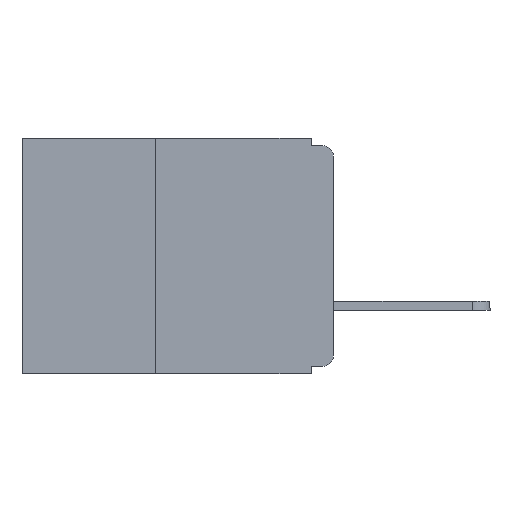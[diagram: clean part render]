
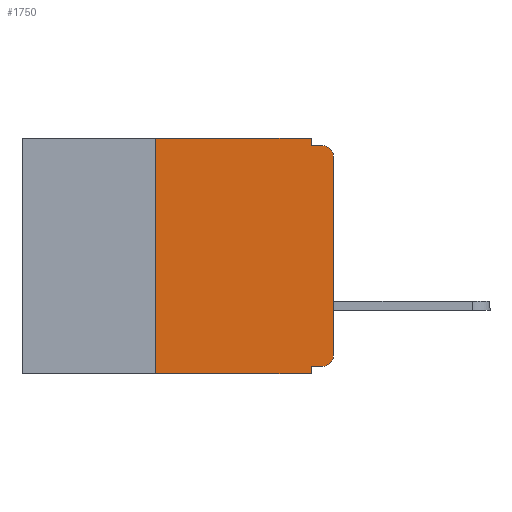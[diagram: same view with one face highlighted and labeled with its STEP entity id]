
A CAD part, left-side view. The second image highlights one B-rep face of the part: STEP entity #1750.
In plain terms, the highlighted planar face has unit normal (-1, 0, 0).
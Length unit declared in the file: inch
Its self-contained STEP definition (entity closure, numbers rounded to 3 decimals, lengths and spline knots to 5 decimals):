
#452 = CARTESIAN_POINT ( 'NONE',  ( 0., 0.031, 0. ) ) ;
#1750 = ADVANCED_FACE ( 'NONE', ( #9253 ), #13834, .F. ) ;
#2847 = EDGE_CURVE ( 'NONE', #5645, #4229, #3118, .T. ) ;
#3118 = CIRCLE ( 'NONE', #18012, 0.015 ) ;
#3281 = VERTEX_POINT ( 'NONE', #8255 ) ;
#3384 = ORIENTED_EDGE ( 'NONE', *, *, #25762, .F. ) ;
#3414 = DIRECTION ( 'NONE',  ( -1., 0., 0. ) ) ;
#4038 = VERTEX_POINT ( 'NONE', #6024 ) ;
#4229 = VERTEX_POINT ( 'NONE', #22526 ) ;
#5309 = VECTOR ( 'NONE', #12262, 39.37008 ) ;
#5504 = EDGE_LOOP ( 'NONE', ( #11152, #24888, #24540, #13641, #25946, #3384, #28102, #7116, #8626, #20961 ) ) ;
#5645 = VERTEX_POINT ( 'NONE', #16124 ) ;
#6024 = CARTESIAN_POINT ( 'NONE',  ( 0., 0.031, 0. ) ) ;
#6256 = VECTOR ( 'NONE', #16753, 39.37008 ) ;
#6316 = CARTESIAN_POINT ( 'NONE',  ( 0., 0.25, -0.33 ) ) ;
#6868 = CARTESIAN_POINT ( 'NONE',  ( 0., 0.437, 0. ) ) ;
#6939 = VERTEX_POINT ( 'NONE', #25939 ) ;
#6987 = LINE ( 'NONE', #23756, #6256 ) ;
#7116 = ORIENTED_EDGE ( 'NONE', *, *, #27860, .F. ) ;
#7436 = CIRCLE ( 'NONE', #28601, 0.015 ) ;
#7560 = VECTOR ( 'NONE', #28402, 39.37008 ) ;
#7600 = VERTEX_POINT ( 'NONE', #27231 ) ;
#7620 = VERTEX_POINT ( 'NONE', #15717 ) ;
#8001 = LINE ( 'NONE', #6316, #13425 ) ;
#8014 = DIRECTION ( 'NONE',  ( 0., 0., -1. ) ) ;
#8255 = CARTESIAN_POINT ( 'NONE',  ( 0., 0., -0.025 ) ) ;
#8626 = ORIENTED_EDGE ( 'NONE', *, *, #26238, .F. ) ;
#8899 = VECTOR ( 'NONE', #28273, 39.37008 ) ;
#9253 = FACE_OUTER_BOUND ( 'NONE', #5504, .T. ) ;
#9616 = EDGE_CURVE ( 'NONE', #24625, #13089, #23746, .T. ) ;
#11152 = ORIENTED_EDGE ( 'NONE', *, *, #16789, .T. ) ;
#11341 = CARTESIAN_POINT ( 'NONE',  ( 0., 0.031, -0.01 ) ) ;
#11606 = DIRECTION ( 'NONE',  ( 0., -1., 0. ) ) ;
#12262 = DIRECTION ( 'NONE',  ( 0., 0., -1. ) ) ;
#12718 = DIRECTION ( 'NONE',  ( 0., 1., 0. ) ) ;
#12784 = EDGE_CURVE ( 'NONE', #4038, #24625, #18439, .T. ) ;
#13089 = VERTEX_POINT ( 'NONE', #17900 ) ;
#13377 = VECTOR ( 'NONE', #29876, 39.37008 ) ;
#13425 = VECTOR ( 'NONE', #24902, 39.37008 ) ;
#13641 = ORIENTED_EDGE ( 'NONE', *, *, #12784, .F. ) ;
#13834 = PLANE ( 'NONE',  #20342 ) ;
#14919 = CARTESIAN_POINT ( 'NONE',  ( 0., 0., -0.32 ) ) ;
#15717 = CARTESIAN_POINT ( 'NONE',  ( 0., 0.25, 0. ) ) ;
#16014 = DIRECTION ( 'NONE',  ( -1., 0., 0. ) ) ;
#16124 = CARTESIAN_POINT ( 'NONE',  ( 0., 0.015, -0.32 ) ) ;
#16564 = EDGE_CURVE ( 'NONE', #7620, #4038, #26407, .T. ) ;
#16753 = DIRECTION ( 'NONE',  ( 0., -1., 0. ) ) ;
#16789 = EDGE_CURVE ( 'NONE', #4229, #3281, #26019, .T. ) ;
#17427 = CARTESIAN_POINT ( 'NONE',  ( 0., 0.015, -0.025 ) ) ;
#17900 = CARTESIAN_POINT ( 'NONE',  ( 0., 0.015, -0.01 ) ) ;
#18012 = AXIS2_PLACEMENT_3D ( 'NONE', #22515, #16014, #8014 ) ;
#18439 = LINE ( 'NONE', #452, #5309 ) ;
#18515 = EDGE_CURVE ( 'NONE', #3281, #13089, #7436, .T. ) ;
#18534 = VECTOR ( 'NONE', #12718, 39.37008 ) ;
#19364 = CARTESIAN_POINT ( 'NONE',  ( 0., 0.25, -0.33 ) ) ;
#19587 = EDGE_CURVE ( 'NONE', #24938, #6939, #6987, .T. ) ;
#19771 = DIRECTION ( 'NONE',  ( 0., 0., -1. ) ) ;
#20342 = AXIS2_PLACEMENT_3D ( 'NONE', #27712, #29252, #21802 ) ;
#20961 = ORIENTED_EDGE ( 'NONE', *, *, #2847, .T. ) ;
#21802 = DIRECTION ( 'NONE',  ( 0., 0., -1. ) ) ;
#22515 = CARTESIAN_POINT ( 'NONE',  ( 0., 0.015, -0.305 ) ) ;
#22526 = CARTESIAN_POINT ( 'NONE',  ( 0., 0., -0.305 ) ) ;
#23746 = LINE ( 'NONE', #29960, #29755 ) ;
#23756 = CARTESIAN_POINT ( 'NONE',  ( 0., 0.437, -0.33 ) ) ;
#24540 = ORIENTED_EDGE ( 'NONE', *, *, #9616, .F. ) ;
#24625 = VERTEX_POINT ( 'NONE', #11341 ) ;
#24694 = LINE ( 'NONE', #14919, #18534 ) ;
#24888 = ORIENTED_EDGE ( 'NONE', *, *, #18515, .T. ) ;
#24902 = DIRECTION ( 'NONE',  ( 0., 0., 1. ) ) ;
#24938 = VERTEX_POINT ( 'NONE', #19364 ) ;
#25762 = EDGE_CURVE ( 'NONE', #24938, #7620, #8001, .T. ) ;
#25939 = CARTESIAN_POINT ( 'NONE',  ( 0., 0.031, -0.33 ) ) ;
#25946 = ORIENTED_EDGE ( 'NONE', *, *, #16564, .F. ) ;
#25977 = CARTESIAN_POINT ( 'NONE',  ( 0., 0.031, -0.33 ) ) ;
#26019 = LINE ( 'NONE', #26103, #7560 ) ;
#26103 = CARTESIAN_POINT ( 'NONE',  ( 0., 0., 0. ) ) ;
#26238 = EDGE_CURVE ( 'NONE', #5645, #7600, #24694, .T. ) ;
#26407 = LINE ( 'NONE', #6868, #13377 ) ;
#27231 = CARTESIAN_POINT ( 'NONE',  ( 0., 0.031, -0.32 ) ) ;
#27316 = LINE ( 'NONE', #25977, #8899 ) ;
#27712 = CARTESIAN_POINT ( 'NONE',  ( 0., 0.437, 0. ) ) ;
#27860 = EDGE_CURVE ( 'NONE', #7600, #6939, #27316, .T. ) ;
#28102 = ORIENTED_EDGE ( 'NONE', *, *, #19587, .T. ) ;
#28273 = DIRECTION ( 'NONE',  ( 0., 0., -1. ) ) ;
#28402 = DIRECTION ( 'NONE',  ( 0., 0., 1. ) ) ;
#28601 = AXIS2_PLACEMENT_3D ( 'NONE', #17427, #3414, #19771 ) ;
#29252 = DIRECTION ( 'NONE',  ( 1., 0., 0. ) ) ;
#29755 = VECTOR ( 'NONE', #11606, 39.37008 ) ;
#29876 = DIRECTION ( 'NONE',  ( 0., -1., 0. ) ) ;
#29960 = CARTESIAN_POINT ( 'NONE',  ( 0., 0., -0.01 ) ) ;
